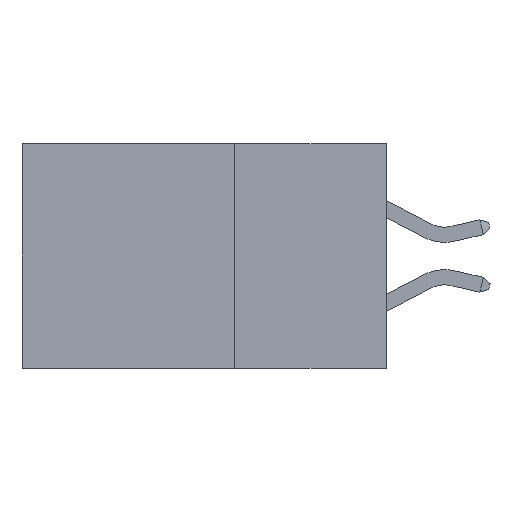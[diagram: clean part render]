
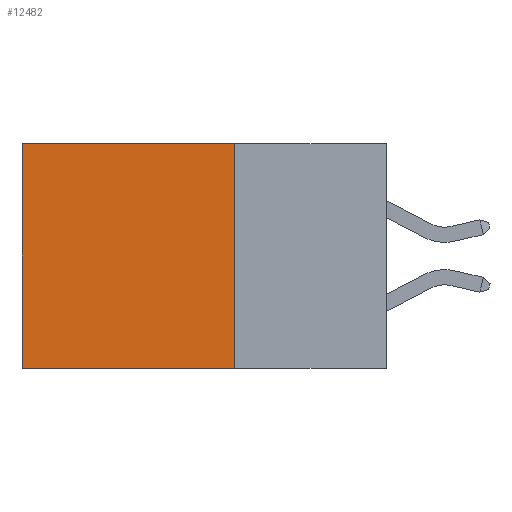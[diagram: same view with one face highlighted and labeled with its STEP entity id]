
A CAD part, left-side view. The second image highlights one B-rep face of the part: STEP entity #12482.
In plain terms, the highlighted planar face has unit normal (-1, 0, 0).
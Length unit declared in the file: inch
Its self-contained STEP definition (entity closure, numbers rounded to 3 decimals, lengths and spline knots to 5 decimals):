
#287 = CARTESIAN_POINT ( 'NONE',  ( 0.298, 0.25, 0. ) ) ;
#415 = CARTESIAN_POINT ( 'NONE',  ( 0.298, 0.6, -0.37 ) ) ;
#457 = CARTESIAN_POINT ( 'NONE',  ( 0.298, 0.25, 0. ) ) ;
#932 = ORIENTED_EDGE ( 'NONE', *, *, #9838, .T. ) ;
#1170 = ORIENTED_EDGE ( 'NONE', *, *, #1962, .T. ) ;
#1962 = EDGE_CURVE ( 'NONE', #4807, #3197, #2219, .T. ) ;
#2219 = LINE ( 'NONE', #287, #11670 ) ;
#2306 = FACE_OUTER_BOUND ( 'NONE', #6653, .T. ) ;
#3197 = VERTEX_POINT ( 'NONE', #15219 ) ;
#3463 = CARTESIAN_POINT ( 'NONE',  ( 0.298, 0.25, -0.37 ) ) ;
#3795 = VECTOR ( 'NONE', #4454, 39.37008 ) ;
#4155 = CARTESIAN_POINT ( 'NONE',  ( 0.298, 0.25, 0. ) ) ;
#4391 = AXIS2_PLACEMENT_3D ( 'NONE', #21132, #6723, #6811 ) ;
#4454 = DIRECTION ( 'NONE',  ( 0., 0., -1. ) ) ;
#4807 = VERTEX_POINT ( 'NONE', #457 ) ;
#5142 = DIRECTION ( 'NONE',  ( 0., 0., -1. ) ) ;
#6653 = EDGE_LOOP ( 'NONE', ( #932, #18896, #19246, #1170 ) ) ;
#6723 = DIRECTION ( 'NONE',  ( 1., 0., 0. ) ) ;
#6811 = DIRECTION ( 'NONE',  ( 0., 0., -1. ) ) ;
#7940 = VECTOR ( 'NONE', #12698, 39.37008 ) ;
#8536 = LINE ( 'NONE', #4155, #3795 ) ;
#9368 = LINE ( 'NONE', #15869, #13242 ) ;
#9838 = EDGE_CURVE ( 'NONE', #3197, #14858, #9368, .T. ) ;
#10495 = EDGE_CURVE ( 'NONE', #16092, #14858, #18241, .T. ) ;
#11670 = VECTOR ( 'NONE', #19533, 39.37008 ) ;
#12482 = ADVANCED_FACE ( 'NONE', ( #2306 ), #18845, .F. ) ;
#12698 = DIRECTION ( 'NONE',  ( 0., 1., 0. ) ) ;
#13242 = VECTOR ( 'NONE', #5142, 39.37008 ) ;
#14858 = VERTEX_POINT ( 'NONE', #415 ) ;
#15219 = CARTESIAN_POINT ( 'NONE',  ( 0.298, 0.6, 0. ) ) ;
#15364 = EDGE_CURVE ( 'NONE', #4807, #16092, #8536, .T. ) ;
#15869 = CARTESIAN_POINT ( 'NONE',  ( 0.298, 0.6, 0. ) ) ;
#16092 = VERTEX_POINT ( 'NONE', #3463 ) ;
#18241 = LINE ( 'NONE', #21411, #7940 ) ;
#18845 = PLANE ( 'NONE',  #4391 ) ;
#18896 = ORIENTED_EDGE ( 'NONE', *, *, #10495, .F. ) ;
#19246 = ORIENTED_EDGE ( 'NONE', *, *, #15364, .F. ) ;
#19533 = DIRECTION ( 'NONE',  ( 0., 1., 0. ) ) ;
#21132 = CARTESIAN_POINT ( 'NONE',  ( 0.298, 0.25, 0. ) ) ;
#21411 = CARTESIAN_POINT ( 'NONE',  ( 0.298, 0.25, -0.37 ) ) ;
